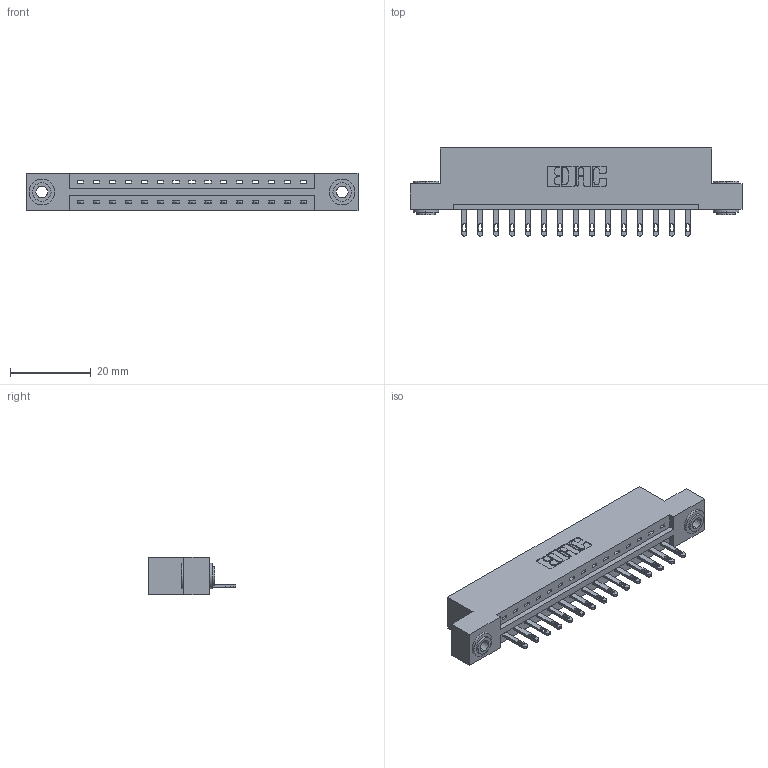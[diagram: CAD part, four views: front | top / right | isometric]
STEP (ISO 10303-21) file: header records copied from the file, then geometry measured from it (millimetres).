
FILE_DESCRIPTION (( 'STEP AP203' ), '1' );
FILE_NAME ('887-015-500-103.STEP', '2020-09-20T16:59:54', ( '' ), ( '' ), 'SwSTEP 2.0', 'SolidWorks 2020', '' );
FILE_SCHEMA (( 'CONFIG_CONTROL_DESIGN' ));
Length unit declared in the file: inch
Products named in the file (4): 887-015-500-103; 345-292-001_345-293-100; 345-250-002_345-250-002-102; 837 Part_Flush Mounting Lugs - 0.156 Dia-TH
Assembly tree (18 placements, depth 2):
  887-015-500-103
    837 Part_Flush Mounting Lugs - 0.156 Dia-TH
    345-292-001_345-293-100  x15
    345-250-002_345-250-002-102  x2
Bounding box: 82.45 x 21.85 x 9.4 mm (x, y, z)
Volume: 8259.9 mm3; surface area: 8653.3 mm2
Topology: 18 solids, 18 shells, 1022 faces, 3087 edges, 2054 vertices
Faces by surface type: plane 680, cylinder 334, cone 8
Entity records: 15222 total; most frequent: CARTESIAN_POINT 2626, ORIENTED_EDGE 2570, DIRECTION 2301, EDGE_CURVE 1285, LINE 1129, VECTOR 1129, VERTEX_POINT 854, AXIS2_PLACEMENT_3D 586
